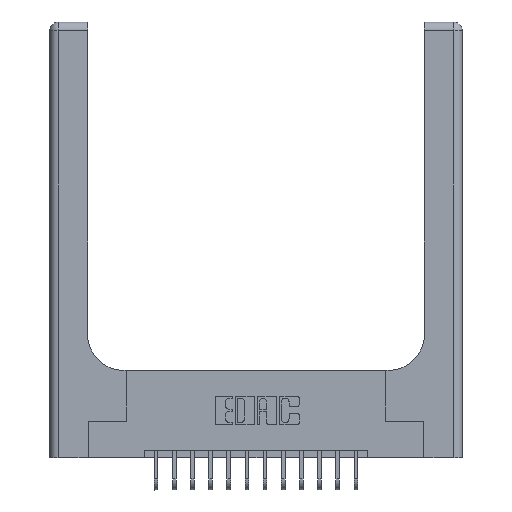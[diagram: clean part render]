
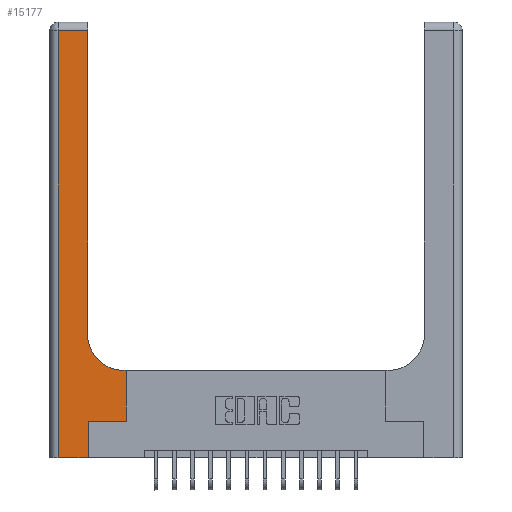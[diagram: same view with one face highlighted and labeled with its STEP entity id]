
A CAD part, top view. The second image highlights one B-rep face of the part: STEP entity #15177.
In plain terms, the highlighted planar face has unit normal (0, 0, 1).
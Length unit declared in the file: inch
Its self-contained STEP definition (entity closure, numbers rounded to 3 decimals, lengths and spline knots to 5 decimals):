
#235 = LINE ( 'NONE', #6211, #15349 ) ;
#400 = VECTOR ( 'NONE', #1969, 39.37008 ) ;
#481 = CARTESIAN_POINT ( 'NONE',  ( 0.26, 0.6, 0.37 ) ) ;
#607 = DIRECTION ( 'NONE',  ( 0., 0., -1. ) ) ;
#613 = ORIENTED_EDGE ( 'NONE', *, *, #5510, .T. ) ;
#617 = CARTESIAN_POINT ( 'NONE',  ( 0.26, 3., 0.37 ) ) ;
#736 = LINE ( 'NONE', #18751, #18604 ) ;
#1114 = CARTESIAN_POINT ( 'NONE',  ( 0.51, 0.85, 0.37 ) ) ;
#1356 = ORIENTED_EDGE ( 'NONE', *, *, #3748, .T. ) ;
#1750 = VERTEX_POINT ( 'NONE', #5670 ) ;
#1753 = LINE ( 'NONE', #481, #18504 ) ;
#1969 = DIRECTION ( 'NONE',  ( 0., 1., 0. ) ) ;
#2167 = DIRECTION ( 'NONE',  ( 0., 1., 0. ) ) ;
#2754 = VERTEX_POINT ( 'NONE', #19042 ) ;
#3235 = ORIENTED_EDGE ( 'NONE', *, *, #18888, .T. ) ;
#3251 = VERTEX_POINT ( 'NONE', #13591 ) ;
#3429 = VECTOR ( 'NONE', #2167, 39.37008 ) ;
#3441 = DIRECTION ( 'NONE',  ( -1., 0., 0. ) ) ;
#3748 = EDGE_CURVE ( 'NONE', #13950, #16728, #14544, .T. ) ;
#4134 = ORIENTED_EDGE ( 'NONE', *, *, #12852, .T. ) ;
#4286 = AXIS2_PLACEMENT_3D ( 'NONE', #8343, #607, #3441 ) ;
#4337 = ORIENTED_EDGE ( 'NONE', *, *, #10369, .T. ) ;
#4630 = VECTOR ( 'NONE', #11803, 39.37008 ) ;
#4686 = CIRCLE ( 'NONE', #7186, 0.25 ) ;
#5510 = EDGE_CURVE ( 'NONE', #2754, #3251, #235, .T. ) ;
#5670 = CARTESIAN_POINT ( 'NONE',  ( 0.51, 0.6, 0.37 ) ) ;
#5809 = DIRECTION ( 'NONE',  ( 1., 0., 0. ) ) ;
#5896 = LINE ( 'NONE', #13063, #4630 ) ;
#6188 = ORIENTED_EDGE ( 'NONE', *, *, #18304, .T. ) ;
#6211 = CARTESIAN_POINT ( 'NONE',  ( 0., 2.94, 0.37 ) ) ;
#6394 = VERTEX_POINT ( 'NONE', #17027 ) ;
#6428 = VECTOR ( 'NONE', #6599, 39.37008 ) ;
#6599 = DIRECTION ( 'NONE',  ( 0., 1., 0. ) ) ;
#6842 = VECTOR ( 'NONE', #10363, 39.37008 ) ;
#6942 = CARTESIAN_POINT ( 'NONE',  ( 0.265, 0.25, 0.37 ) ) ;
#7186 = AXIS2_PLACEMENT_3D ( 'NONE', #1114, #17804, #5809 ) ;
#7394 = EDGE_LOOP ( 'NONE', ( #4134, #613, #10737, #15381, #3235, #1356, #16707, #4337, #6188 ) ) ;
#7763 = LINE ( 'NONE', #13737, #400 ) ;
#8343 = CARTESIAN_POINT ( 'NONE',  ( 0., 3., 0.37 ) ) ;
#8445 = EDGE_CURVE ( 'NONE', #16728, #12248, #7763, .T. ) ;
#9078 = CARTESIAN_POINT ( 'NONE',  ( 0.26, 0.85, 0.37 ) ) ;
#9549 = VERTEX_POINT ( 'NONE', #9078 ) ;
#10279 = CARTESIAN_POINT ( 'NONE',  ( 0.265, 0.25, 0.37 ) ) ;
#10363 = DIRECTION ( 'NONE',  ( 1., 0., 0. ) ) ;
#10369 = EDGE_CURVE ( 'NONE', #12248, #1750, #1753, .T. ) ;
#10737 = ORIENTED_EDGE ( 'NONE', *, *, #16190, .T. ) ;
#11528 = VERTEX_POINT ( 'NONE', #14834 ) ;
#11803 = DIRECTION ( 'NONE',  ( 0., -1., 0. ) ) ;
#12248 = VERTEX_POINT ( 'NONE', #13230 ) ;
#12760 = FACE_OUTER_BOUND ( 'NONE', #7394, .T. ) ;
#12852 = EDGE_CURVE ( 'NONE', #9549, #2754, #15372, .T. ) ;
#13063 = CARTESIAN_POINT ( 'NONE',  ( 0.06, 3., 0.37 ) ) ;
#13230 = CARTESIAN_POINT ( 'NONE',  ( 0.528, 0.6, 0.37 ) ) ;
#13591 = CARTESIAN_POINT ( 'NONE',  ( 0.06, 2.94, 0.37 ) ) ;
#13737 = CARTESIAN_POINT ( 'NONE',  ( 0.528, 0.25, 0.37 ) ) ;
#13950 = VERTEX_POINT ( 'NONE', #6942 ) ;
#14544 = LINE ( 'NONE', #10279, #6842 ) ;
#14834 = CARTESIAN_POINT ( 'NONE',  ( 0.265, 0., 0.37 ) ) ;
#15177 = ADVANCED_FACE ( 'NONE', ( #12760 ), #18632, .F. ) ;
#15184 = DIRECTION ( 'NONE',  ( -1., 0., 0. ) ) ;
#15337 = DIRECTION ( 'NONE',  ( -1., 0., 0. ) ) ;
#15349 = VECTOR ( 'NONE', #15184, 39.37008 ) ;
#15372 = LINE ( 'NONE', #617, #6428 ) ;
#15381 = ORIENTED_EDGE ( 'NONE', *, *, #16115, .T. ) ;
#15448 = LINE ( 'NONE', #15540, #3429 ) ;
#15479 = DIRECTION ( 'NONE',  ( 1., 0., 0. ) ) ;
#15540 = CARTESIAN_POINT ( 'NONE',  ( 0.265, 0., 0.37 ) ) ;
#16115 = EDGE_CURVE ( 'NONE', #6394, #11528, #736, .T. ) ;
#16190 = EDGE_CURVE ( 'NONE', #3251, #6394, #5896, .T. ) ;
#16707 = ORIENTED_EDGE ( 'NONE', *, *, #8445, .T. ) ;
#16728 = VERTEX_POINT ( 'NONE', #17460 ) ;
#17027 = CARTESIAN_POINT ( 'NONE',  ( 0.06, 0., 0.37 ) ) ;
#17460 = CARTESIAN_POINT ( 'NONE',  ( 0.528, 0.25, 0.37 ) ) ;
#17804 = DIRECTION ( 'NONE',  ( 0., 0., -1. ) ) ;
#18304 = EDGE_CURVE ( 'NONE', #1750, #9549, #4686, .T. ) ;
#18504 = VECTOR ( 'NONE', #15337, 39.37008 ) ;
#18604 = VECTOR ( 'NONE', #15479, 39.37008 ) ;
#18632 = PLANE ( 'NONE',  #4286 ) ;
#18751 = CARTESIAN_POINT ( 'NONE',  ( 0., 0., 0.37 ) ) ;
#18888 = EDGE_CURVE ( 'NONE', #11528, #13950, #15448, .T. ) ;
#19042 = CARTESIAN_POINT ( 'NONE',  ( 0.26, 2.94, 0.37 ) ) ;
